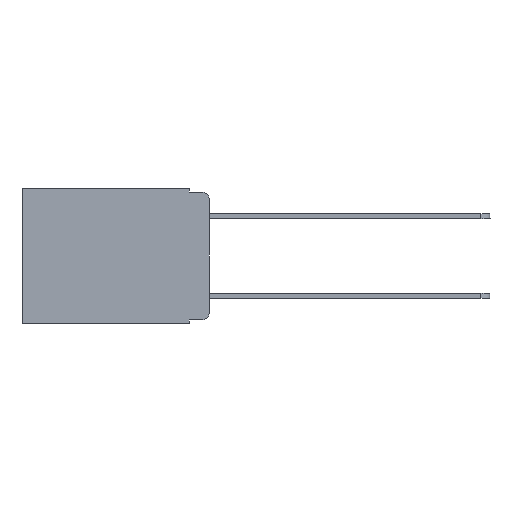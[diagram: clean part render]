
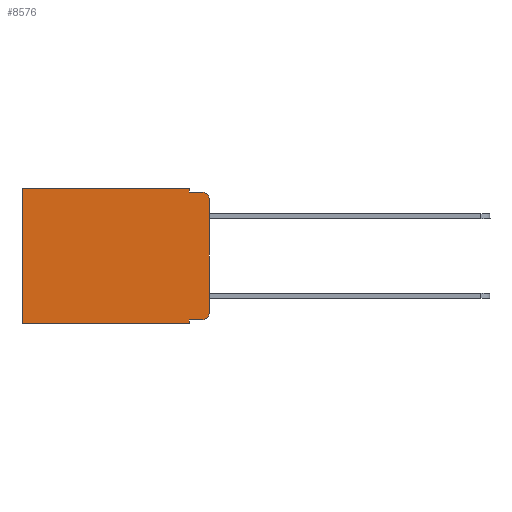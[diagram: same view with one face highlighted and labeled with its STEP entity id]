
A CAD part, left-side view. The second image highlights one B-rep face of the part: STEP entity #8576.
In plain terms, the highlighted planar face has unit normal (-1, 0, 0).
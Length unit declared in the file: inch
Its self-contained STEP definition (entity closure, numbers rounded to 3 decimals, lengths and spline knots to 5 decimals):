
#19 = DIRECTION ( 'NONE',  ( 0., 0., -1. ) ) ;
#31 = VECTOR ( 'NONE', #6527, 39.37008 ) ;
#129 = EDGE_CURVE ( 'NONE', #4186, #760, #8960, .T. ) ;
#168 = VECTOR ( 'NONE', #1403, 39.37008 ) ;
#297 = EDGE_LOOP ( 'NONE', ( #5151, #5628, #8326, #6629, #6529, #7308, #3723, #2462, #726, #1225 ) ) ;
#309 = DIRECTION ( 'NONE',  ( 0., 1., 0. ) ) ;
#386 = CARTESIAN_POINT ( 'NONE',  ( 0.298, 0.02, -0.01 ) ) ;
#598 = EDGE_CURVE ( 'NONE', #760, #3431, #2764, .T. ) ;
#625 = AXIS2_PLACEMENT_3D ( 'NONE', #3039, #5906, #19 ) ;
#726 = ORIENTED_EDGE ( 'NONE', *, *, #4773, .T. ) ;
#760 = VERTEX_POINT ( 'NONE', #6147 ) ;
#827 = VECTOR ( 'NONE', #2384, 39.37008 ) ;
#955 = EDGE_CURVE ( 'NONE', #3501, #6359, #8493, .T. ) ;
#1017 = EDGE_CURVE ( 'NONE', #2970, #2378, #1269, .T. ) ;
#1225 = ORIENTED_EDGE ( 'NONE', *, *, #6144, .T. ) ;
#1269 = LINE ( 'NONE', #9392, #31 ) ;
#1403 = DIRECTION ( 'NONE',  ( 0., 0., -1. ) ) ;
#1562 = DIRECTION ( 'NONE',  ( 0., 0., -1. ) ) ;
#1625 = CARTESIAN_POINT ( 'NONE',  ( 0.298, 0., 0. ) ) ;
#2154 = CARTESIAN_POINT ( 'NONE',  ( 0.298, 0.051, -0.343 ) ) ;
#2182 = DIRECTION ( 'NONE',  ( -1., 0., 0. ) ) ;
#2289 = CARTESIAN_POINT ( 'NONE',  ( 0.298, 0.051, -0.333 ) ) ;
#2378 = VERTEX_POINT ( 'NONE', #6611 ) ;
#2384 = DIRECTION ( 'NONE',  ( 0., 0., -1. ) ) ;
#2462 = ORIENTED_EDGE ( 'NONE', *, *, #5501, .F. ) ;
#2533 = CARTESIAN_POINT ( 'NONE',  ( 0.298, 0.051, -0.333 ) ) ;
#2602 = DIRECTION ( 'NONE',  ( 0., -1., 0. ) ) ;
#2764 = LINE ( 'NONE', #7472, #827 ) ;
#2970 = VERTEX_POINT ( 'NONE', #3718 ) ;
#3039 = CARTESIAN_POINT ( 'NONE',  ( 0.298, 0.02, -0.03 ) ) ;
#3109 = LINE ( 'NONE', #5244, #3925 ) ;
#3431 = VERTEX_POINT ( 'NONE', #7176 ) ;
#3496 = AXIS2_PLACEMENT_3D ( 'NONE', #7273, #2182, #8129 ) ;
#3501 = VERTEX_POINT ( 'NONE', #4052 ) ;
#3676 = LINE ( 'NONE', #4591, #4143 ) ;
#3718 = CARTESIAN_POINT ( 'NONE',  ( 0.298, 0., -0.03 ) ) ;
#3723 = ORIENTED_EDGE ( 'NONE', *, *, #6930, .F. ) ;
#3851 = VECTOR ( 'NONE', #5460, 39.37008 ) ;
#3925 = VECTOR ( 'NONE', #1562, 39.37008 ) ;
#3981 = LINE ( 'NONE', #2289, #3851 ) ;
#4038 = VECTOR ( 'NONE', #2602, 39.37008 ) ;
#4052 = CARTESIAN_POINT ( 'NONE',  ( 0.298, 0.051, -0.01 ) ) ;
#4143 = VECTOR ( 'NONE', #5364, 39.37008 ) ;
#4186 = VERTEX_POINT ( 'NONE', #7992 ) ;
#4340 = CARTESIAN_POINT ( 'NONE',  ( 0.298, 0.051, 0. ) ) ;
#4379 = CIRCLE ( 'NONE', #625, 0.02 ) ;
#4591 = CARTESIAN_POINT ( 'NONE',  ( 0.298, 0., -0.343 ) ) ;
#4674 = EDGE_CURVE ( 'NONE', #2970, #6359, #4379, .T. ) ;
#4773 = EDGE_CURVE ( 'NONE', #9335, #6829, #3981, .T. ) ;
#5151 = ORIENTED_EDGE ( 'NONE', *, *, #1017, .F. ) ;
#5244 = CARTESIAN_POINT ( 'NONE',  ( 0.298, 0.051, 0. ) ) ;
#5364 = DIRECTION ( 'NONE',  ( 0., 1., 0. ) ) ;
#5460 = DIRECTION ( 'NONE',  ( 0., -1., 0. ) ) ;
#5501 = EDGE_CURVE ( 'NONE', #9335, #9005, #8626, .T. ) ;
#5628 = ORIENTED_EDGE ( 'NONE', *, *, #4674, .T. ) ;
#5733 = FACE_OUTER_BOUND ( 'NONE', #297, .T. ) ;
#5906 = DIRECTION ( 'NONE',  ( -1., 0., 0. ) ) ;
#6144 = EDGE_CURVE ( 'NONE', #6829, #2378, #8501, .T. ) ;
#6147 = CARTESIAN_POINT ( 'NONE',  ( 0.298, 0.473, 0. ) ) ;
#6243 = EDGE_CURVE ( 'NONE', #4186, #3501, #3109, .T. ) ;
#6359 = VERTEX_POINT ( 'NONE', #386 ) ;
#6527 = DIRECTION ( 'NONE',  ( 0., 0., -1. ) ) ;
#6529 = ORIENTED_EDGE ( 'NONE', *, *, #129, .T. ) ;
#6611 = CARTESIAN_POINT ( 'NONE',  ( 0.298, 0., -0.313 ) ) ;
#6629 = ORIENTED_EDGE ( 'NONE', *, *, #6243, .F. ) ;
#6775 = DIRECTION ( 'NONE',  ( 1., 0., 0. ) ) ;
#6829 = VERTEX_POINT ( 'NONE', #8737 ) ;
#6835 = PLANE ( 'NONE',  #8285 ) ;
#6930 = EDGE_CURVE ( 'NONE', #9005, #3431, #3676, .T. ) ;
#7176 = CARTESIAN_POINT ( 'NONE',  ( 0.298, 0.473, -0.343 ) ) ;
#7273 = CARTESIAN_POINT ( 'NONE',  ( 0.298, 0.02, -0.313 ) ) ;
#7308 = ORIENTED_EDGE ( 'NONE', *, *, #598, .T. ) ;
#7472 = CARTESIAN_POINT ( 'NONE',  ( 0.298, 0.473, 0. ) ) ;
#7552 = DIRECTION ( 'NONE',  ( 0., 0., -1. ) ) ;
#7992 = CARTESIAN_POINT ( 'NONE',  ( 0.298, 0.051, 0. ) ) ;
#8129 = DIRECTION ( 'NONE',  ( 0., 0., -1. ) ) ;
#8285 = AXIS2_PLACEMENT_3D ( 'NONE', #1625, #6775, #7552 ) ;
#8326 = ORIENTED_EDGE ( 'NONE', *, *, #955, .F. ) ;
#8354 = CARTESIAN_POINT ( 'NONE',  ( 0.298, 0., 0. ) ) ;
#8493 = LINE ( 'NONE', #8557, #4038 ) ;
#8501 = CIRCLE ( 'NONE', #3496, 0.02 ) ;
#8557 = CARTESIAN_POINT ( 'NONE',  ( 0.298, 0.051, -0.01 ) ) ;
#8576 = ADVANCED_FACE ( 'NONE', ( #5733 ), #6835, .F. ) ;
#8614 = VECTOR ( 'NONE', #309, 39.37008 ) ;
#8626 = LINE ( 'NONE', #4340, #168 ) ;
#8737 = CARTESIAN_POINT ( 'NONE',  ( 0.298, 0.02, -0.333 ) ) ;
#8960 = LINE ( 'NONE', #8354, #8614 ) ;
#9005 = VERTEX_POINT ( 'NONE', #2154 ) ;
#9335 = VERTEX_POINT ( 'NONE', #2533 ) ;
#9392 = CARTESIAN_POINT ( 'NONE',  ( 0.298, 0., 0. ) ) ;
